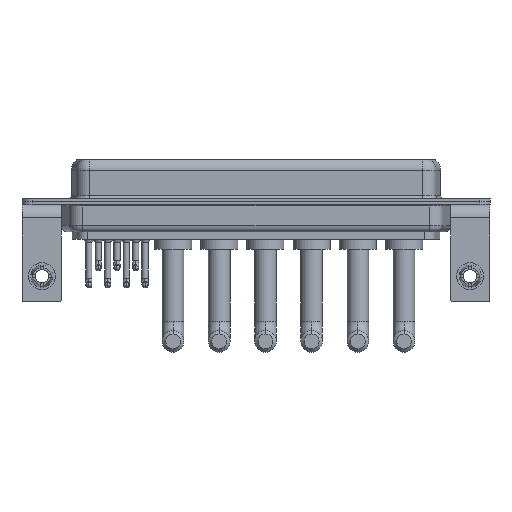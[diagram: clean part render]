
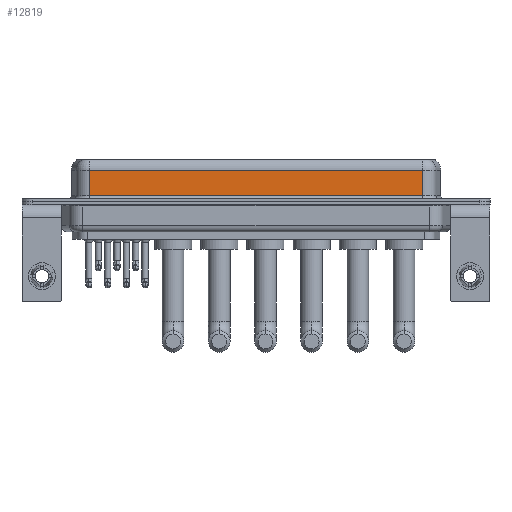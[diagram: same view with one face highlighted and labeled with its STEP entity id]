
A CAD part, front view. The second image highlights one B-rep face of the part: STEP entity #12819.
In plain terms, the highlighted planar face has unit normal (0, -1, 0).
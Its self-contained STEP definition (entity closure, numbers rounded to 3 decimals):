
#10 = LINE ( 'NONE', #5172, #7709 ) ;
#405 = VERTEX_POINT ( 'NONE', #4312 ) ;
#3385 = LINE ( 'NONE', #19511, #4979 ) ;
#4312 = CARTESIAN_POINT ( 'NONE',  ( 56.462, -3.95, 4.65 ) ) ;
#4704 = LINE ( 'NONE', #11139, #5460 ) ;
#4979 = VECTOR ( 'NONE', #12912, 1000. ) ;
#5172 = CARTESIAN_POINT ( 'NONE',  ( 56.462, -3.95, 0.9 ) ) ;
#5460 = VECTOR ( 'NONE', #17563, 1000. ) ;
#5864 = FACE_OUTER_BOUND ( 'NONE', #15804, .T. ) ;
#7106 = LINE ( 'NONE', #13528, #16906 ) ;
#7184 = CARTESIAN_POINT ( 'NONE',  ( 7.038, -3.95, 0.9 ) ) ;
#7256 = EDGE_CURVE ( 'NONE', #405, #15487, #4704, .T. ) ;
#7700 = CARTESIAN_POINT ( 'NONE',  ( 56.462, -3.95, 0.9 ) ) ;
#7709 = VECTOR ( 'NONE', #10027, 1000. ) ;
#8756 = EDGE_CURVE ( 'NONE', #15487, #17679, #7106, .T. ) ;
#9024 = DIRECTION ( 'NONE',  ( 0., 0., 1. ) ) ;
#10027 = DIRECTION ( 'NONE',  ( 1., 0., 0. ) ) ;
#11139 = CARTESIAN_POINT ( 'NONE',  ( 56.462, -3.95, 4.65 ) ) ;
#12819 = ADVANCED_FACE ( 'NONE', ( #5864 ), #14178, .F. ) ;
#12912 = DIRECTION ( 'NONE',  ( 0., 0., -1. ) ) ;
#13119 = DIRECTION ( 'NONE',  ( 0., 0., -1. ) ) ;
#13528 = CARTESIAN_POINT ( 'NONE',  ( 7.038, -3.95, 6.4 ) ) ;
#14178 = PLANE ( 'NONE',  #19398 ) ;
#15350 = EDGE_CURVE ( 'NONE', #405, #16435, #3385, .T. ) ;
#15462 = ORIENTED_EDGE ( 'NONE', *, *, #8756, .T. ) ;
#15487 = VERTEX_POINT ( 'NONE', #18361 ) ;
#15804 = EDGE_LOOP ( 'NONE', ( #17464, #17918, #15462, #20500 ) ) ;
#16146 = EDGE_CURVE ( 'NONE', #17679, #16435, #10, .T. ) ;
#16435 = VERTEX_POINT ( 'NONE', #7700 ) ;
#16906 = VECTOR ( 'NONE', #13119, 1000. ) ;
#17452 = DIRECTION ( 'NONE',  ( 0., 1., 0. ) ) ;
#17464 = ORIENTED_EDGE ( 'NONE', *, *, #15350, .F. ) ;
#17563 = DIRECTION ( 'NONE',  ( -1., 0., 0. ) ) ;
#17679 = VERTEX_POINT ( 'NONE', #7184 ) ;
#17918 = ORIENTED_EDGE ( 'NONE', *, *, #7256, .T. ) ;
#18361 = CARTESIAN_POINT ( 'NONE',  ( 7.038, -3.95, 4.65 ) ) ;
#18705 = CARTESIAN_POINT ( 'NONE',  ( 56.462, -3.95, 6.4 ) ) ;
#19398 = AXIS2_PLACEMENT_3D ( 'NONE', #18705, #17452, #9024 ) ;
#19511 = CARTESIAN_POINT ( 'NONE',  ( 56.462, -3.95, 6.4 ) ) ;
#20500 = ORIENTED_EDGE ( 'NONE', *, *, #16146, .T. ) ;
